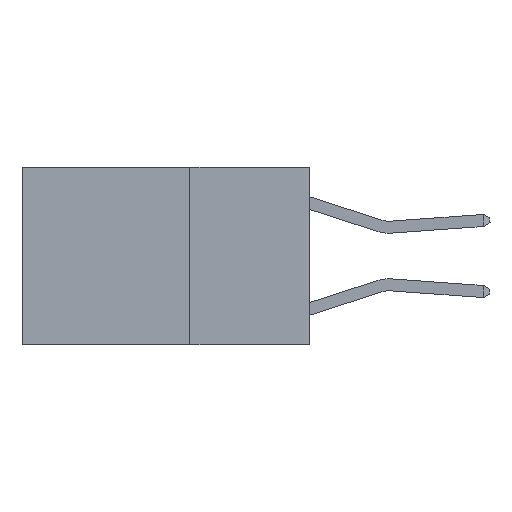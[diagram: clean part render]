
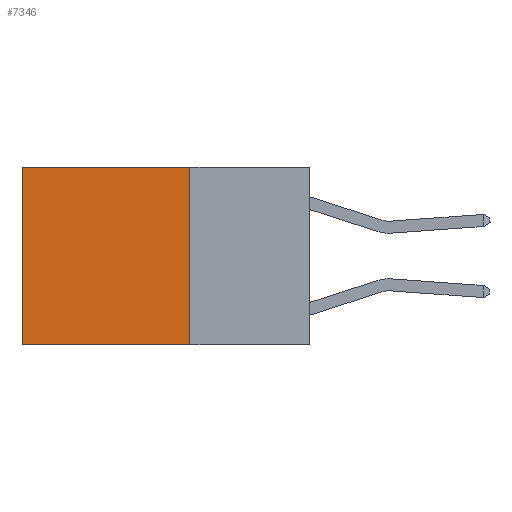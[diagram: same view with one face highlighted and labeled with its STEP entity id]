
A CAD part, left-side view. The second image highlights one B-rep face of the part: STEP entity #7346.
In plain terms, the highlighted planar face has unit normal (-1, 0, 0).
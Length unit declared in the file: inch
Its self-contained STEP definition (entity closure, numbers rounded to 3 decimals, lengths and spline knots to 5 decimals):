
#26 = DIRECTION ( 'NONE',  ( 0., 0., -1. ) ) ;
#335 = ORIENTED_EDGE ( 'NONE', *, *, #1293, .T. ) ;
#406 = EDGE_CURVE ( 'NONE', #6007, #9378, #14419, .T. ) ;
#923 = EDGE_CURVE ( 'NONE', #13668, #7572, #2769, .T. ) ;
#1293 = EDGE_CURVE ( 'NONE', #13668, #6007, #2200, .T. ) ;
#2200 = LINE ( 'NONE', #4230, #12784 ) ;
#2769 = LINE ( 'NONE', #12462, #11345 ) ;
#3673 = DIRECTION ( 'NONE',  ( 0., 1., 0. ) ) ;
#4075 = AXIS2_PLACEMENT_3D ( 'NONE', #13983, #7009, #26 ) ;
#4230 = CARTESIAN_POINT ( 'NONE',  ( 0.2625, 0.25, 0. ) ) ;
#4887 = DIRECTION ( 'NONE',  ( 0., 0., -1. ) ) ;
#5836 = PLANE ( 'NONE',  #4075 ) ;
#6007 = VERTEX_POINT ( 'NONE', #9456 ) ;
#6913 = ORIENTED_EDGE ( 'NONE', *, *, #406, .T. ) ;
#7009 = DIRECTION ( 'NONE',  ( 1., 0., 0. ) ) ;
#7346 = ADVANCED_FACE ( 'NONE', ( #11050 ), #5836, .F. ) ;
#7572 = VERTEX_POINT ( 'NONE', #8556 ) ;
#7573 = ORIENTED_EDGE ( 'NONE', *, *, #9255, .F. ) ;
#7601 = ORIENTED_EDGE ( 'NONE', *, *, #923, .F. ) ;
#8556 = CARTESIAN_POINT ( 'NONE',  ( 0.2625, 0.25, -0.37 ) ) ;
#8610 = VECTOR ( 'NONE', #4887, 39.37008 ) ;
#8975 = DIRECTION ( 'NONE',  ( 0., 1., 0. ) ) ;
#9038 = EDGE_LOOP ( 'NONE', ( #6913, #7573, #7601, #335 ) ) ;
#9255 = EDGE_CURVE ( 'NONE', #7572, #9378, #12801, .T. ) ;
#9378 = VERTEX_POINT ( 'NONE', #13832 ) ;
#9456 = CARTESIAN_POINT ( 'NONE',  ( 0.2625, 0.6, 0. ) ) ;
#9704 = VECTOR ( 'NONE', #8975, 39.37008 ) ;
#10067 = CARTESIAN_POINT ( 'NONE',  ( 0.2625, 0.25, 0. ) ) ;
#11050 = FACE_OUTER_BOUND ( 'NONE', #9038, .T. ) ;
#11345 = VECTOR ( 'NONE', #12348, 39.37008 ) ;
#12348 = DIRECTION ( 'NONE',  ( 0., 0., -1. ) ) ;
#12462 = CARTESIAN_POINT ( 'NONE',  ( 0.2625, 0.25, 0. ) ) ;
#12784 = VECTOR ( 'NONE', #3673, 39.37008 ) ;
#12801 = LINE ( 'NONE', #13596, #9704 ) ;
#13596 = CARTESIAN_POINT ( 'NONE',  ( 0.2625, 0.25, -0.37 ) ) ;
#13668 = VERTEX_POINT ( 'NONE', #10067 ) ;
#13815 = CARTESIAN_POINT ( 'NONE',  ( 0.2625, 0.6, 0. ) ) ;
#13832 = CARTESIAN_POINT ( 'NONE',  ( 0.2625, 0.6, -0.37 ) ) ;
#13983 = CARTESIAN_POINT ( 'NONE',  ( 0.2625, 0.25, 0. ) ) ;
#14419 = LINE ( 'NONE', #13815, #8610 ) ;
